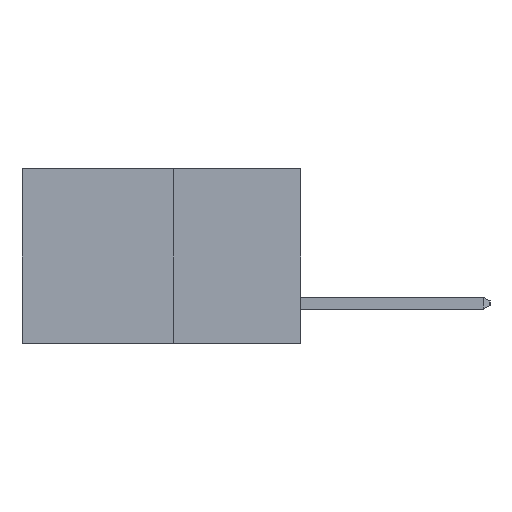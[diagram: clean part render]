
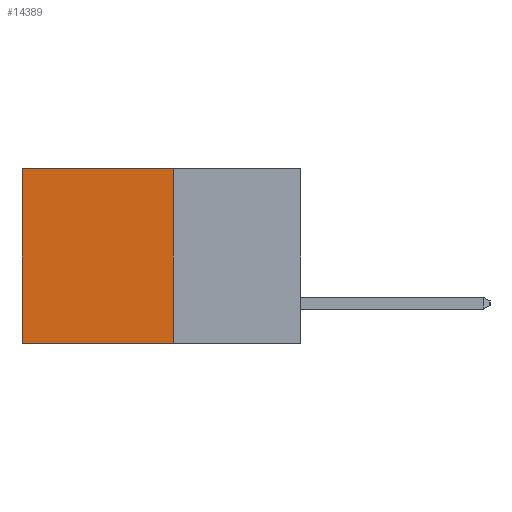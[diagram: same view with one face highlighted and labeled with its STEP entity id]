
A CAD part, left-side view. The second image highlights one B-rep face of the part: STEP entity #14389.
In plain terms, the highlighted planar face has unit normal (-1, 0, 0).
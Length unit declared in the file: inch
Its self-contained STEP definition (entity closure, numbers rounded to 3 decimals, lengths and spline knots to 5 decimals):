
#972 = EDGE_CURVE ( 'NONE', #15056, #3796, #12450, .T. ) ;
#1295 = AXIS2_PLACEMENT_3D ( 'NONE', #12165, #5882, #14655 ) ;
#1615 = VERTEX_POINT ( 'NONE', #11493 ) ;
#1661 = DIRECTION ( 'NONE',  ( 0., 0., -1. ) ) ;
#1779 = CARTESIAN_POINT ( 'NONE',  ( 0.277, 0.27, -0.37 ) ) ;
#2978 = CARTESIAN_POINT ( 'NONE',  ( 0.277, 0.27, 0. ) ) ;
#3614 = ORIENTED_EDGE ( 'NONE', *, *, #12623, .T. ) ;
#3796 = VERTEX_POINT ( 'NONE', #4410 ) ;
#4304 = DIRECTION ( 'NONE',  ( 0., 1., 0. ) ) ;
#4410 = CARTESIAN_POINT ( 'NONE',  ( 0.277, 0.59, -0.37 ) ) ;
#4485 = EDGE_CURVE ( 'NONE', #1615, #3796, #11349, .T. ) ;
#4553 = PLANE ( 'NONE',  #1295 ) ;
#4815 = DIRECTION ( 'NONE',  ( 0., 1., 0. ) ) ;
#5552 = LINE ( 'NONE', #2978, #11872 ) ;
#5882 = DIRECTION ( 'NONE',  ( 1., 0., 0. ) ) ;
#6181 = CARTESIAN_POINT ( 'NONE',  ( 0.277, 0.27, -0.37 ) ) ;
#7274 = EDGE_LOOP ( 'NONE', ( #8410, #8821, #12951, #3614 ) ) ;
#8000 = VERTEX_POINT ( 'NONE', #8803 ) ;
#8410 = ORIENTED_EDGE ( 'NONE', *, *, #4485, .T. ) ;
#8477 = EDGE_CURVE ( 'NONE', #8000, #15056, #12276, .T. ) ;
#8803 = CARTESIAN_POINT ( 'NONE',  ( 0.277, 0.27, 0. ) ) ;
#8821 = ORIENTED_EDGE ( 'NONE', *, *, #972, .F. ) ;
#10060 = DIRECTION ( 'NONE',  ( 0., 0., -1. ) ) ;
#10393 = CARTESIAN_POINT ( 'NONE',  ( 0.277, 0.59, -0.37 ) ) ;
#10899 = VECTOR ( 'NONE', #4815, 39.37008 ) ;
#10953 = CARTESIAN_POINT ( 'NONE',  ( 0.277, 0.27, -0.37 ) ) ;
#11349 = LINE ( 'NONE', #10393, #14659 ) ;
#11493 = CARTESIAN_POINT ( 'NONE',  ( 0.277, 0.59, 0. ) ) ;
#11872 = VECTOR ( 'NONE', #4304, 39.37008 ) ;
#12165 = CARTESIAN_POINT ( 'NONE',  ( 0.277, 0.27, -0.37 ) ) ;
#12276 = LINE ( 'NONE', #1779, #15944 ) ;
#12450 = LINE ( 'NONE', #6181, #10899 ) ;
#12623 = EDGE_CURVE ( 'NONE', #8000, #1615, #5552, .T. ) ;
#12951 = ORIENTED_EDGE ( 'NONE', *, *, #8477, .F. ) ;
#14389 = ADVANCED_FACE ( 'NONE', ( #16422 ), #4553, .F. ) ;
#14655 = DIRECTION ( 'NONE',  ( 0., 0., -1. ) ) ;
#14659 = VECTOR ( 'NONE', #10060, 39.37008 ) ;
#15056 = VERTEX_POINT ( 'NONE', #10953 ) ;
#15944 = VECTOR ( 'NONE', #1661, 39.37008 ) ;
#16422 = FACE_OUTER_BOUND ( 'NONE', #7274, .T. ) ;
